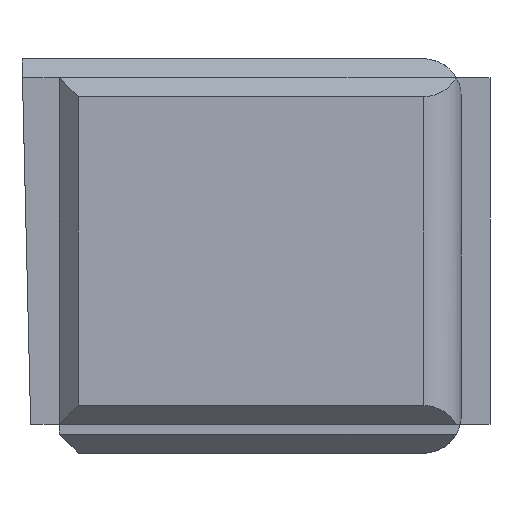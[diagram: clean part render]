
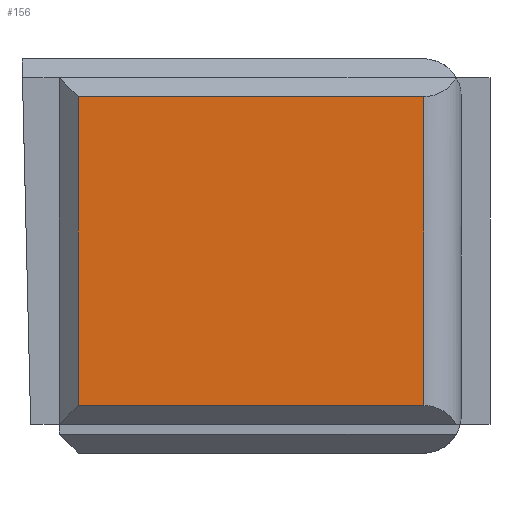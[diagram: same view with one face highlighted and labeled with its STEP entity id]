
A CAD part, front view. The second image highlights one B-rep face of the part: STEP entity #156.
In plain terms, the highlighted planar face has unit normal (0, -1, 0).
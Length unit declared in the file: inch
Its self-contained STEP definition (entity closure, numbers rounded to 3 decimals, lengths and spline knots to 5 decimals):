
#90 = EDGE_CURVE ( 'NONE', #343, #384, #1094, .T. ) ;
#91 = EDGE_CURVE ( 'NONE', #341, #407, #1079, .T. ) ;
#95 = EDGE_CURVE ( 'NONE', #384, #341, #1088, .T. ) ;
#98 = EDGE_CURVE ( 'NONE', #407, #343, #1091, .T. ) ;
#156 = ADVANCED_FACE ( 'NONE', ( #434 ), #734, .F. ) ;
#204 = ORIENTED_EDGE ( 'NONE', *, *, #91, .T. ) ;
#205 = ORIENTED_EDGE ( 'NONE', *, *, #90, .T. ) ;
#226 = ORIENTED_EDGE ( 'NONE', *, *, #95, .T. ) ;
#230 = ORIENTED_EDGE ( 'NONE', *, *, #98, .T. ) ;
#341 = VERTEX_POINT ( 'NONE', #806 ) ;
#343 = VERTEX_POINT ( 'NONE', #836 ) ;
#384 = VERTEX_POINT ( 'NONE', #829 ) ;
#407 = VERTEX_POINT ( 'NONE', #1257 ) ;
#422 = AXIS2_PLACEMENT_3D ( 'NONE', #731, #720, #726 ) ;
#434 = FACE_OUTER_BOUND ( 'NONE', #933, .T. ) ;
#569 = VECTOR ( 'NONE', #1093, 39.37008 ) ;
#575 = VECTOR ( 'NONE', #1101, 39.37008 ) ;
#576 = VECTOR ( 'NONE', #1103, 39.37008 ) ;
#577 = VECTOR ( 'NONE', #1100, 39.37008 ) ;
#720 = DIRECTION ( 'NONE',  ( 0., 1., 0. ) ) ;
#726 = DIRECTION ( 'NONE',  ( 0., 0., 1. ) ) ;
#731 = CARTESIAN_POINT ( 'NONE',  ( 0., -0.3, 0. ) ) ;
#734 = PLANE ( 'NONE',  #422 ) ;
#806 = CARTESIAN_POINT ( 'NONE',  ( 4.19454, -0.3, -3.62087 ) ) ;
#829 = CARTESIAN_POINT ( 'NONE',  ( 0.58748, -0.3, -3.62087 ) ) ;
#836 = CARTESIAN_POINT ( 'NONE',  ( 0.58748, -0.3, -0.3937 ) ) ;
#933 = EDGE_LOOP ( 'NONE', ( #226, #204, #230, #205 ) ) ;
#1079 = LINE ( 'NONE', #1102, #575 ) ;
#1080 = CARTESIAN_POINT ( 'NONE',  ( 0., -0.3, -3.62087 ) ) ;
#1081 = CARTESIAN_POINT ( 'NONE',  ( 0.58748, -0.3, 0. ) ) ;
#1088 = LINE ( 'NONE', #1080, #577 ) ;
#1091 = LINE ( 'NONE', #1092, #569 ) ;
#1092 = CARTESIAN_POINT ( 'NONE',  ( 0., -0.3, -0.3937 ) ) ;
#1093 = DIRECTION ( 'NONE',  ( -1., 0., 0. ) ) ;
#1094 = LINE ( 'NONE', #1081, #576 ) ;
#1100 = DIRECTION ( 'NONE',  ( 1., 0., 0. ) ) ;
#1101 = DIRECTION ( 'NONE',  ( 0., 0., 1. ) ) ;
#1102 = CARTESIAN_POINT ( 'NONE',  ( 4.19454, -0.3, -0.3937 ) ) ;
#1103 = DIRECTION ( 'NONE',  ( 0., 0., -1. ) ) ;
#1257 = CARTESIAN_POINT ( 'NONE',  ( 4.19454, -0.3, -0.3937 ) ) ;
